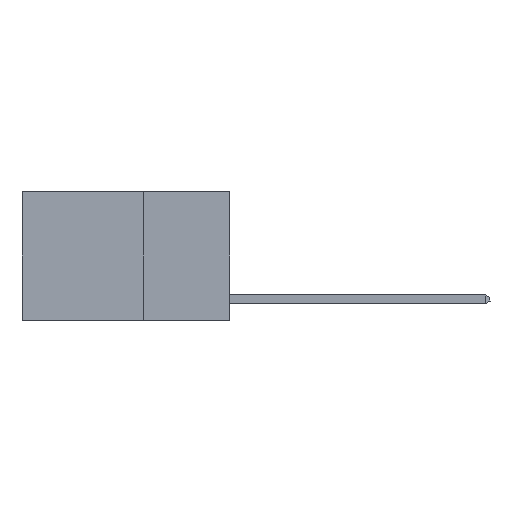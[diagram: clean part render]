
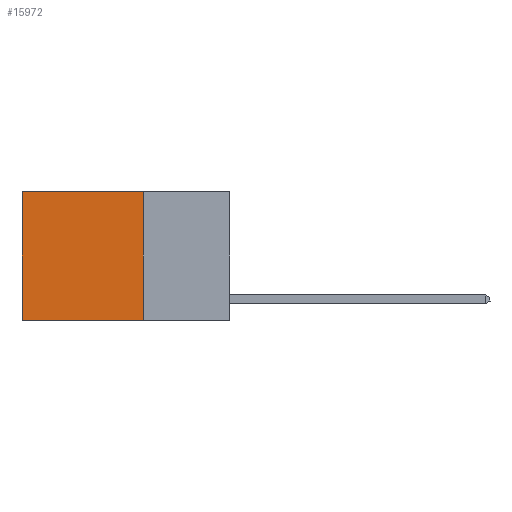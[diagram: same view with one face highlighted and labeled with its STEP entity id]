
A CAD part, left-side view. The second image highlights one B-rep face of the part: STEP entity #15972.
In plain terms, the highlighted planar face has unit normal (-1, 0, 0).
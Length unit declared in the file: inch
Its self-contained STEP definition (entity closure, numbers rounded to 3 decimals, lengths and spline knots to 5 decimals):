
#597 = FACE_OUTER_BOUND ( 'NONE', #9616, .T. ) ;
#996 = VECTOR ( 'NONE', #6037, 39.37008 ) ;
#1009 = CARTESIAN_POINT ( 'NONE',  ( 0.2625, 0.25, 0. ) ) ;
#1497 = CARTESIAN_POINT ( 'NONE',  ( 0.2625, 0.25, -0.37 ) ) ;
#2049 = CARTESIAN_POINT ( 'NONE',  ( 0.2625, 0.25, 0. ) ) ;
#2537 = LINE ( 'NONE', #1497, #6673 ) ;
#2573 = CARTESIAN_POINT ( 'NONE',  ( 0.2625, 0.25, 0. ) ) ;
#2815 = VECTOR ( 'NONE', #12584, 39.37008 ) ;
#2834 = EDGE_CURVE ( 'NONE', #15697, #16330, #8884, .T. ) ;
#3345 = CARTESIAN_POINT ( 'NONE',  ( 0.2625, 0.25, -0.37 ) ) ;
#3648 = VECTOR ( 'NONE', #4451, 39.37008 ) ;
#4038 = VERTEX_POINT ( 'NONE', #10107 ) ;
#4184 = AXIS2_PLACEMENT_3D ( 'NONE', #9827, #7149, #14756 ) ;
#4451 = DIRECTION ( 'NONE',  ( 0., 0., -1. ) ) ;
#4735 = PLANE ( 'NONE',  #4184 ) ;
#5317 = EDGE_CURVE ( 'NONE', #15697, #4038, #11753, .T. ) ;
#5808 = ORIENTED_EDGE ( 'NONE', *, *, #11043, .F. ) ;
#6037 = DIRECTION ( 'NONE',  ( 0., 0., -1. ) ) ;
#6673 = VECTOR ( 'NONE', #7874, 39.37008 ) ;
#6748 = EDGE_CURVE ( 'NONE', #4038, #14757, #11583, .T. ) ;
#7149 = DIRECTION ( 'NONE',  ( 1., 0., 0. ) ) ;
#7874 = DIRECTION ( 'NONE',  ( 0., 1., 0. ) ) ;
#8884 = LINE ( 'NONE', #1009, #996 ) ;
#8950 = ORIENTED_EDGE ( 'NONE', *, *, #5317, .T. ) ;
#9616 = EDGE_LOOP ( 'NONE', ( #11594, #5808, #13351, #8950 ) ) ;
#9827 = CARTESIAN_POINT ( 'NONE',  ( 0.2625, 0.25, 0. ) ) ;
#9894 = CARTESIAN_POINT ( 'NONE',  ( 0.2625, 0.6, -0.37 ) ) ;
#10107 = CARTESIAN_POINT ( 'NONE',  ( 0.2625, 0.6, 0. ) ) ;
#11043 = EDGE_CURVE ( 'NONE', #16330, #14757, #2537, .T. ) ;
#11583 = LINE ( 'NONE', #12065, #3648 ) ;
#11594 = ORIENTED_EDGE ( 'NONE', *, *, #6748, .T. ) ;
#11753 = LINE ( 'NONE', #2573, #2815 ) ;
#12065 = CARTESIAN_POINT ( 'NONE',  ( 0.2625, 0.6, 0. ) ) ;
#12584 = DIRECTION ( 'NONE',  ( 0., 1., 0. ) ) ;
#13351 = ORIENTED_EDGE ( 'NONE', *, *, #2834, .F. ) ;
#14756 = DIRECTION ( 'NONE',  ( 0., 0., -1. ) ) ;
#14757 = VERTEX_POINT ( 'NONE', #9894 ) ;
#15697 = VERTEX_POINT ( 'NONE', #2049 ) ;
#15972 = ADVANCED_FACE ( 'NONE', ( #597 ), #4735, .F. ) ;
#16330 = VERTEX_POINT ( 'NONE', #3345 ) ;
